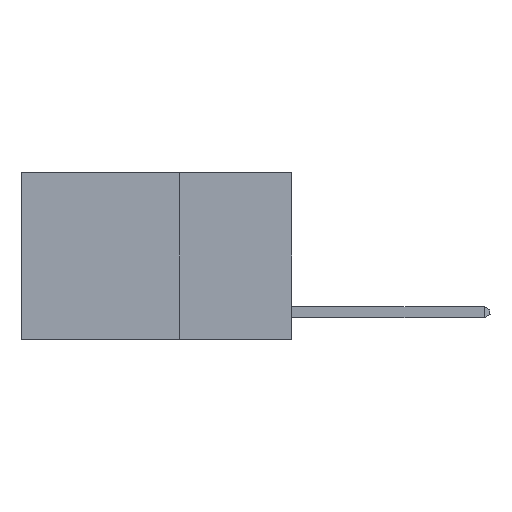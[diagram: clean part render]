
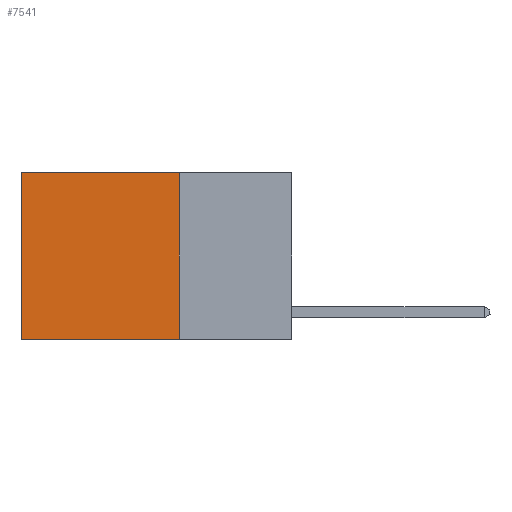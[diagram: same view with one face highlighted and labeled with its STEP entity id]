
A CAD part, left-side view. The second image highlights one B-rep face of the part: STEP entity #7541.
In plain terms, the highlighted planar face has unit normal (-1, 0, 0).
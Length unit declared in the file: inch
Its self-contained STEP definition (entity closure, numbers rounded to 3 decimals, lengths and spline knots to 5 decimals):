
#37 = AXIS2_PLACEMENT_3D ( 'NONE', #12300, #12429, #20645 ) ;
#622 = DIRECTION ( 'NONE',  ( 0., 0., -1. ) ) ;
#623 = VERTEX_POINT ( 'NONE', #24931 ) ;
#1767 = EDGE_CURVE ( 'NONE', #623, #4396, #19856, .T. ) ;
#1843 = VECTOR ( 'NONE', #2486, 39.37008 ) ;
#2486 = DIRECTION ( 'NONE',  ( 0., 1., 0. ) ) ;
#2892 = CARTESIAN_POINT ( 'NONE',  ( 0.2625, 0.6, -0.37 ) ) ;
#3236 = ORIENTED_EDGE ( 'NONE', *, *, #19151, .T. ) ;
#3369 = VECTOR ( 'NONE', #5576, 39.37008 ) ;
#3752 = VERTEX_POINT ( 'NONE', #10027 ) ;
#4396 = VERTEX_POINT ( 'NONE', #2892 ) ;
#5576 = DIRECTION ( 'NONE',  ( 0., 0., -1. ) ) ;
#6301 = VECTOR ( 'NONE', #8568, 39.37008 ) ;
#7541 = ADVANCED_FACE ( 'NONE', ( #16586 ), #16707, .F. ) ;
#8180 = CARTESIAN_POINT ( 'NONE',  ( 0.2625, 0.25, 0. ) ) ;
#8568 = DIRECTION ( 'NONE',  ( 0., 1., 0. ) ) ;
#9373 = CARTESIAN_POINT ( 'NONE',  ( 0.2625, 0.6, 0. ) ) ;
#10027 = CARTESIAN_POINT ( 'NONE',  ( 0.2625, 0.25, 0. ) ) ;
#10120 = LINE ( 'NONE', #8180, #6301 ) ;
#12300 = CARTESIAN_POINT ( 'NONE',  ( 0.2625, 0.25, 0. ) ) ;
#12429 = DIRECTION ( 'NONE',  ( 1., 0., 0. ) ) ;
#13529 = LINE ( 'NONE', #9373, #3369 ) ;
#13906 = ORIENTED_EDGE ( 'NONE', *, *, #23689, .T. ) ;
#14383 = CARTESIAN_POINT ( 'NONE',  ( 0.2625, 0.25, -0.37 ) ) ;
#16543 = CARTESIAN_POINT ( 'NONE',  ( 0.2625, 0.25, 0. ) ) ;
#16586 = FACE_OUTER_BOUND ( 'NONE', #23983, .T. ) ;
#16707 = PLANE ( 'NONE',  #37 ) ;
#17632 = EDGE_CURVE ( 'NONE', #3752, #623, #18633, .T. ) ;
#18633 = LINE ( 'NONE', #16543, #19175 ) ;
#19151 = EDGE_CURVE ( 'NONE', #23817, #4396, #13529, .T. ) ;
#19175 = VECTOR ( 'NONE', #622, 39.37008 ) ;
#19856 = LINE ( 'NONE', #14383, #1843 ) ;
#20645 = DIRECTION ( 'NONE',  ( 0., 0., -1. ) ) ;
#22828 = ORIENTED_EDGE ( 'NONE', *, *, #17632, .F. ) ;
#23689 = EDGE_CURVE ( 'NONE', #3752, #23817, #10120, .T. ) ;
#23817 = VERTEX_POINT ( 'NONE', #24980 ) ;
#23983 = EDGE_LOOP ( 'NONE', ( #3236, #24486, #22828, #13906 ) ) ;
#24486 = ORIENTED_EDGE ( 'NONE', *, *, #1767, .F. ) ;
#24931 = CARTESIAN_POINT ( 'NONE',  ( 0.2625, 0.25, -0.37 ) ) ;
#24980 = CARTESIAN_POINT ( 'NONE',  ( 0.2625, 0.6, 0. ) ) ;
